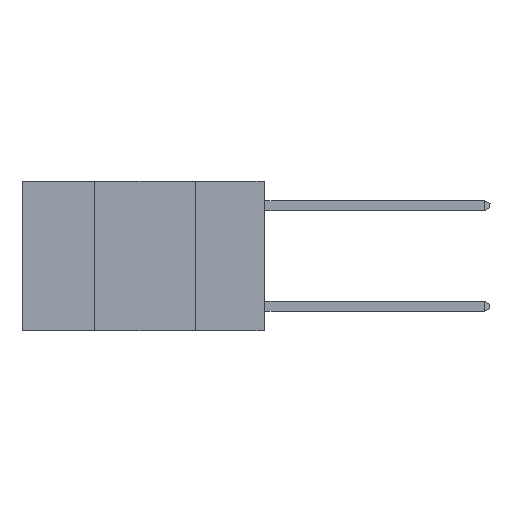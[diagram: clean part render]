
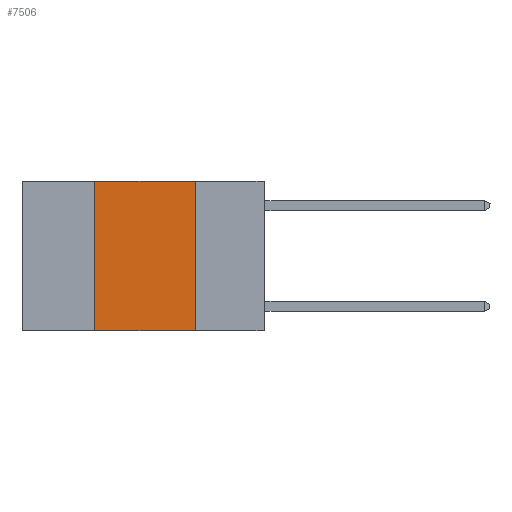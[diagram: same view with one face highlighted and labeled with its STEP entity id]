
A CAD part, left-side view. The second image highlights one B-rep face of the part: STEP entity #7506.
In plain terms, the highlighted planar face has unit normal (-1, 0, 0).
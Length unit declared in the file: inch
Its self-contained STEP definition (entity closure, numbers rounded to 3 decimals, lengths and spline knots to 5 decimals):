
#125 = LINE ( 'NONE', #514, #1183 ) ;
#456 = LINE ( 'NONE', #3085, #5859 ) ;
#514 = CARTESIAN_POINT ( 'NONE',  ( 0., 0.6, 0. ) ) ;
#635 = EDGE_CURVE ( 'NONE', #8383, #8253, #7079, .T. ) ;
#655 = AXIS2_PLACEMENT_3D ( 'NONE', #1663, #5032, #7481 ) ;
#714 = VECTOR ( 'NONE', #6462, 39.37008 ) ;
#1054 = VECTOR ( 'NONE', #8431, 39.37008 ) ;
#1183 = VECTOR ( 'NONE', #3148, 39.37008 ) ;
#1216 = CARTESIAN_POINT ( 'NONE',  ( 0., 0.17, 0. ) ) ;
#1663 = CARTESIAN_POINT ( 'NONE',  ( 0., 0.6, 0. ) ) ;
#2512 = EDGE_CURVE ( 'NONE', #8477, #8253, #456, .T. ) ;
#2783 = ORIENTED_EDGE ( 'NONE', *, *, #4604, .F. ) ;
#3085 = CARTESIAN_POINT ( 'NONE',  ( 0., 0.6, -0.37 ) ) ;
#3148 = DIRECTION ( 'NONE',  ( 0., -1., 0. ) ) ;
#3172 = CARTESIAN_POINT ( 'NONE',  ( 0., 0.42, 0. ) ) ;
#4296 = EDGE_CURVE ( 'NONE', #6317, #8383, #125, .T. ) ;
#4604 = EDGE_CURVE ( 'NONE', #8477, #6317, #6432, .T. ) ;
#5032 = DIRECTION ( 'NONE',  ( 1., 0., 0. ) ) ;
#5083 = PLANE ( 'NONE',  #655 ) ;
#5346 = DIRECTION ( 'NONE',  ( 0., -1., 0. ) ) ;
#5558 = CARTESIAN_POINT ( 'NONE',  ( 0., 0.42, -0.37 ) ) ;
#5859 = VECTOR ( 'NONE', #5346, 39.37008 ) ;
#6153 = ORIENTED_EDGE ( 'NONE', *, *, #635, .F. ) ;
#6276 = FACE_OUTER_BOUND ( 'NONE', #7082, .T. ) ;
#6317 = VERTEX_POINT ( 'NONE', #7204 ) ;
#6432 = LINE ( 'NONE', #3172, #1054 ) ;
#6462 = DIRECTION ( 'NONE',  ( 0., 0., -1. ) ) ;
#6702 = CARTESIAN_POINT ( 'NONE',  ( 0., 0.17, 0. ) ) ;
#7040 = ORIENTED_EDGE ( 'NONE', *, *, #2512, .T. ) ;
#7079 = LINE ( 'NONE', #1216, #714 ) ;
#7082 = EDGE_LOOP ( 'NONE', ( #6153, #7384, #2783, #7040 ) ) ;
#7204 = CARTESIAN_POINT ( 'NONE',  ( 0., 0.42, 0. ) ) ;
#7384 = ORIENTED_EDGE ( 'NONE', *, *, #4296, .F. ) ;
#7481 = DIRECTION ( 'NONE',  ( 0., 0., -1. ) ) ;
#7506 = ADVANCED_FACE ( 'NONE', ( #6276 ), #5083, .F. ) ;
#8253 = VERTEX_POINT ( 'NONE', #8370 ) ;
#8370 = CARTESIAN_POINT ( 'NONE',  ( 0., 0.17, -0.37 ) ) ;
#8383 = VERTEX_POINT ( 'NONE', #6702 ) ;
#8431 = DIRECTION ( 'NONE',  ( 0., 0., 1. ) ) ;
#8477 = VERTEX_POINT ( 'NONE', #5558 ) ;
